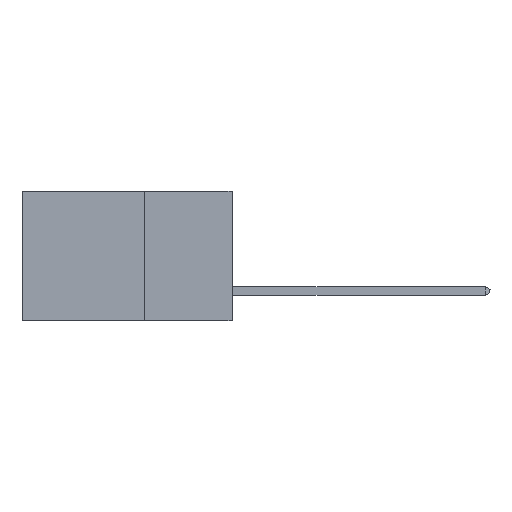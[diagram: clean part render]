
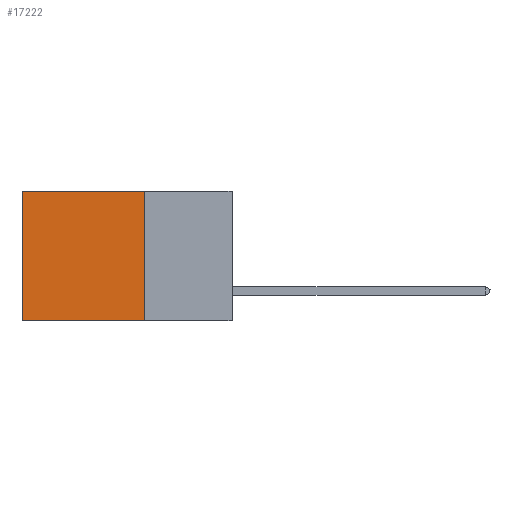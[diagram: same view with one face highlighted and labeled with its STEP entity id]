
A CAD part, left-side view. The second image highlights one B-rep face of the part: STEP entity #17222.
In plain terms, the highlighted planar face has unit normal (-1, 0, 0).
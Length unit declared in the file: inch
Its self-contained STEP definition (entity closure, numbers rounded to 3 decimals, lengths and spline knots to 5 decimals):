
#2 = DIRECTION ( 'NONE',  ( 0., 0., -1. ) ) ;
#1209 = DIRECTION ( 'NONE',  ( 0., 0., -1. ) ) ;
#1859 = DIRECTION ( 'NONE',  ( 0., 1., 0. ) ) ;
#2186 = DIRECTION ( 'NONE',  ( 0., 1., 0. ) ) ;
#2461 = VECTOR ( 'NONE', #2186, 39.37008 ) ;
#2952 = CARTESIAN_POINT ( 'NONE',  ( 0.2875, 0.6, 0. ) ) ;
#3164 = DIRECTION ( 'NONE',  ( 1., 0., 0. ) ) ;
#3870 = FACE_OUTER_BOUND ( 'NONE', #7223, .T. ) ;
#4307 = VERTEX_POINT ( 'NONE', #5623 ) ;
#4418 = ORIENTED_EDGE ( 'NONE', *, *, #9852, .F. ) ;
#4450 = VECTOR ( 'NONE', #16937, 39.37008 ) ;
#4867 = ORIENTED_EDGE ( 'NONE', *, *, #17036, .T. ) ;
#4868 = VERTEX_POINT ( 'NONE', #7026 ) ;
#4889 = VERTEX_POINT ( 'NONE', #2952 ) ;
#5215 = CARTESIAN_POINT ( 'NONE',  ( 0.2875, 0.25, -0.37 ) ) ;
#5468 = LINE ( 'NONE', #18375, #2461 ) ;
#5623 = CARTESIAN_POINT ( 'NONE',  ( 0.2875, 0.25, 0. ) ) ;
#6365 = EDGE_CURVE ( 'NONE', #12563, #4868, #18712, .T. ) ;
#7026 = CARTESIAN_POINT ( 'NONE',  ( 0.2875, 0.6, -0.37 ) ) ;
#7223 = EDGE_LOOP ( 'NONE', ( #10841, #11444, #4418, #4867 ) ) ;
#8816 = CARTESIAN_POINT ( 'NONE',  ( 0.2875, 0.6, 0. ) ) ;
#9852 = EDGE_CURVE ( 'NONE', #4307, #12563, #18584, .T. ) ;
#9970 = AXIS2_PLACEMENT_3D ( 'NONE', #12039, #3164, #2 ) ;
#10405 = VECTOR ( 'NONE', #1859, 39.37008 ) ;
#10841 = ORIENTED_EDGE ( 'NONE', *, *, #11139, .T. ) ;
#11139 = EDGE_CURVE ( 'NONE', #4889, #4868, #15101, .T. ) ;
#11444 = ORIENTED_EDGE ( 'NONE', *, *, #6365, .F. ) ;
#12039 = CARTESIAN_POINT ( 'NONE',  ( 0.2875, 0.25, 0. ) ) ;
#12563 = VERTEX_POINT ( 'NONE', #5215 ) ;
#14181 = VECTOR ( 'NONE', #1209, 39.37008 ) ;
#14856 = PLANE ( 'NONE',  #9970 ) ;
#15101 = LINE ( 'NONE', #8816, #14181 ) ;
#15132 = CARTESIAN_POINT ( 'NONE',  ( 0.2875, 0.25, -0.37 ) ) ;
#15138 = CARTESIAN_POINT ( 'NONE',  ( 0.2875, 0.25, 0. ) ) ;
#16937 = DIRECTION ( 'NONE',  ( 0., 0., -1. ) ) ;
#17036 = EDGE_CURVE ( 'NONE', #4307, #4889, #5468, .T. ) ;
#17222 = ADVANCED_FACE ( 'NONE', ( #3870 ), #14856, .F. ) ;
#18375 = CARTESIAN_POINT ( 'NONE',  ( 0.2875, 0.25, 0. ) ) ;
#18584 = LINE ( 'NONE', #15138, #4450 ) ;
#18712 = LINE ( 'NONE', #15132, #10405 ) ;
